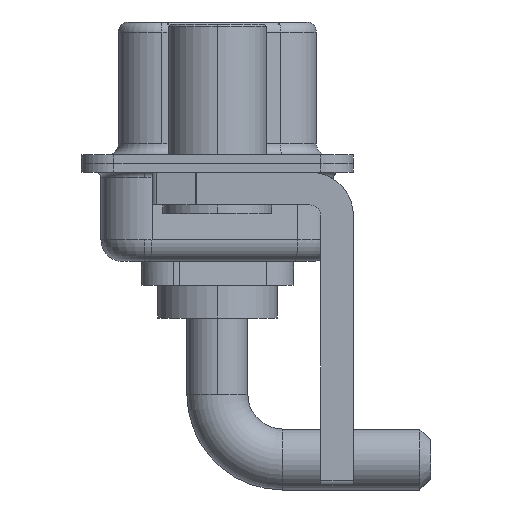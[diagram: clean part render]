
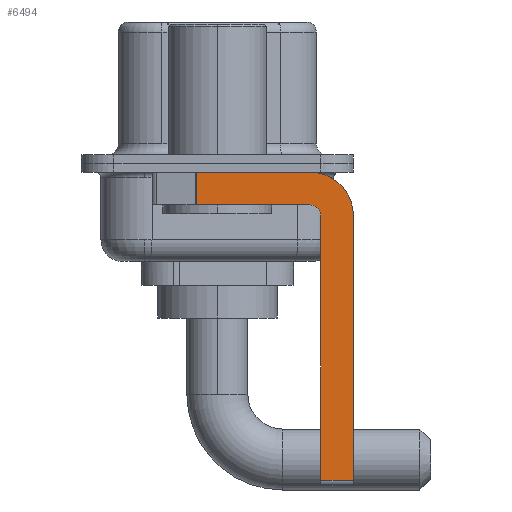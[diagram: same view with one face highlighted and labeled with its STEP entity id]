
A CAD part, left-side view. The second image highlights one B-rep face of the part: STEP entity #6494.
In plain terms, the highlighted planar face has unit normal (-1, 0, 0).
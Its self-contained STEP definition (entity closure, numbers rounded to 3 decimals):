
#143 = CARTESIAN_POINT ( 'NONE',  ( -2.9, 0.978, -1.9 ) ) ;
#235 = CARTESIAN_POINT ( 'NONE',  ( -2.9, -6.25, -2.4 ) ) ;
#439 = CARTESIAN_POINT ( 'NONE',  ( -2.9, -4.25, -2.4 ) ) ;
#512 = VECTOR ( 'NONE', #11714, 1000. ) ;
#1241 = EDGE_CURVE ( 'NONE', #18547, #4208, #15327, .T. ) ;
#1989 = CIRCLE ( 'NONE', #2274, 2. ) ;
#2274 = AXIS2_PLACEMENT_3D ( 'NONE', #439, #10411, #16245 ) ;
#2500 = DIRECTION ( 'NONE',  ( 0., 0., 1. ) ) ;
#3003 = CARTESIAN_POINT ( 'NONE',  ( -2.9, -4.75, -2.4 ) ) ;
#3010 = AXIS2_PLACEMENT_3D ( 'NONE', #18578, #17166, #15936 ) ;
#3390 = VERTEX_POINT ( 'NONE', #13220 ) ;
#3775 = DIRECTION ( 'NONE',  ( 0., -1., 0. ) ) ;
#3927 = EDGE_LOOP ( 'NONE', ( #5653, #5287, #10632, #5885, #12704, #16437, #17406, #16955 ) ) ;
#4208 = VERTEX_POINT ( 'NONE', #14230 ) ;
#4940 = CARTESIAN_POINT ( 'NONE',  ( -2.9, -4.25, -1.9 ) ) ;
#5287 = ORIENTED_EDGE ( 'NONE', *, *, #17396, .T. ) ;
#5556 = DIRECTION ( 'NONE',  ( -1., 0., 0. ) ) ;
#5653 = ORIENTED_EDGE ( 'NONE', *, *, #11922, .F. ) ;
#5885 = ORIENTED_EDGE ( 'NONE', *, *, #9628, .F. ) ;
#6494 = ADVANCED_FACE ( 'NONE', ( #11617 ), #17355, .F. ) ;
#6641 = LINE ( 'NONE', #12390, #10889 ) ;
#6935 = VERTEX_POINT ( 'NONE', #3003 ) ;
#7775 = CARTESIAN_POINT ( 'NONE',  ( -2.9, -6.25, -2.4 ) ) ;
#7867 = CARTESIAN_POINT ( 'NONE',  ( -2.9, -4.75, -14.55 ) ) ;
#8881 = VECTOR ( 'NONE', #2500, 1000. ) ;
#9028 = VERTEX_POINT ( 'NONE', #4940 ) ;
#9628 = EDGE_CURVE ( 'NONE', #6935, #9028, #18364, .T. ) ;
#9949 = AXIS2_PLACEMENT_3D ( 'NONE', #12698, #5556, #12790 ) ;
#10411 = DIRECTION ( 'NONE',  ( 1., 0., 0. ) ) ;
#10632 = ORIENTED_EDGE ( 'NONE', *, *, #17905, .F. ) ;
#10889 = VECTOR ( 'NONE', #13891, 1000. ) ;
#11306 = VECTOR ( 'NONE', #15031, 1000. ) ;
#11347 = VECTOR ( 'NONE', #11696, 1000. ) ;
#11478 = VERTEX_POINT ( 'NONE', #15700 ) ;
#11617 = FACE_OUTER_BOUND ( 'NONE', #3927, .T. ) ;
#11696 = DIRECTION ( 'NONE',  ( 0., 1., 0. ) ) ;
#11714 = DIRECTION ( 'NONE',  ( 0., 0., -1. ) ) ;
#11922 = EDGE_CURVE ( 'NONE', #3390, #11478, #6641, .T. ) ;
#12120 = VERTEX_POINT ( 'NONE', #143 ) ;
#12390 = CARTESIAN_POINT ( 'NONE',  ( -2.9, 3., -0.4 ) ) ;
#12698 = CARTESIAN_POINT ( 'NONE',  ( -2.9, -4.25, -2.4 ) ) ;
#12704 = ORIENTED_EDGE ( 'NONE', *, *, #15953, .F. ) ;
#12726 = LINE ( 'NONE', #17259, #11347 ) ;
#12790 = DIRECTION ( 'NONE',  ( 0., 0., 1. ) ) ;
#13117 = CARTESIAN_POINT ( 'NONE',  ( -2.9, 0.978, -1.9 ) ) ;
#13220 = CARTESIAN_POINT ( 'NONE',  ( -2.9, 0.978, -0.4 ) ) ;
#13520 = LINE ( 'NONE', #7775, #11306 ) ;
#13699 = CARTESIAN_POINT ( 'NONE',  ( -2.9, -4.75, -14.8 ) ) ;
#13891 = DIRECTION ( 'NONE',  ( 0., -1., 0. ) ) ;
#14230 = CARTESIAN_POINT ( 'NONE',  ( -2.9, -6.25, -14.55 ) ) ;
#14529 = VECTOR ( 'NONE', #3775, 1000. ) ;
#15031 = DIRECTION ( 'NONE',  ( 0., 0., -1. ) ) ;
#15292 = LINE ( 'NONE', #13699, #8881 ) ;
#15327 = LINE ( 'NONE', #16747, #14529 ) ;
#15700 = CARTESIAN_POINT ( 'NONE',  ( -2.9, -4.25, -0.4 ) ) ;
#15902 = EDGE_CURVE ( 'NONE', #11478, #17419, #1989, .T. ) ;
#15936 = DIRECTION ( 'NONE',  ( 0., 0., -1. ) ) ;
#15953 = EDGE_CURVE ( 'NONE', #18547, #6935, #15292, .T. ) ;
#16245 = DIRECTION ( 'NONE',  ( 0., 0., -1. ) ) ;
#16437 = ORIENTED_EDGE ( 'NONE', *, *, #1241, .T. ) ;
#16747 = CARTESIAN_POINT ( 'NONE',  ( -2.9, -4.25, -14.55 ) ) ;
#16955 = ORIENTED_EDGE ( 'NONE', *, *, #15902, .F. ) ;
#17166 = DIRECTION ( 'NONE',  ( 1., 0., 0. ) ) ;
#17259 = CARTESIAN_POINT ( 'NONE',  ( -2.9, -4.25, -1.9 ) ) ;
#17355 = PLANE ( 'NONE',  #3010 ) ;
#17396 = EDGE_CURVE ( 'NONE', #3390, #12120, #18226, .T. ) ;
#17406 = ORIENTED_EDGE ( 'NONE', *, *, #18517, .F. ) ;
#17419 = VERTEX_POINT ( 'NONE', #235 ) ;
#17905 = EDGE_CURVE ( 'NONE', #9028, #12120, #12726, .T. ) ;
#18226 = LINE ( 'NONE', #13117, #512 ) ;
#18364 = CIRCLE ( 'NONE', #9949, 0.5 ) ;
#18517 = EDGE_CURVE ( 'NONE', #17419, #4208, #13520, .T. ) ;
#18547 = VERTEX_POINT ( 'NONE', #7867 ) ;
#18578 = CARTESIAN_POINT ( 'NONE',  ( -2.9, -4.25, -2.4 ) ) ;
